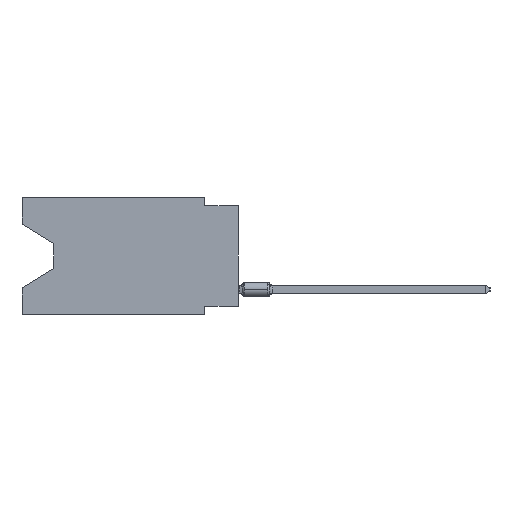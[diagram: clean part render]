
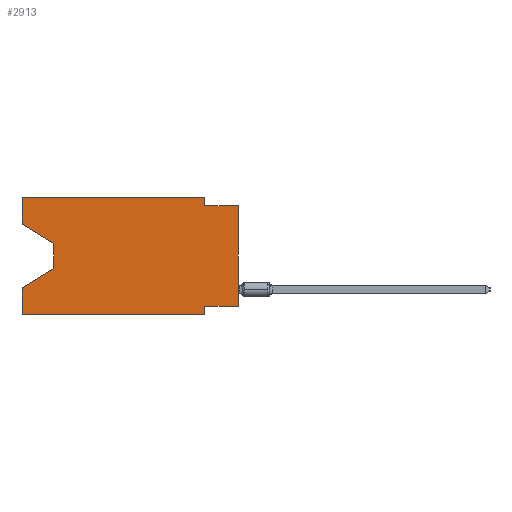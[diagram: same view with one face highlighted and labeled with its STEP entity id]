
A CAD part, left-side view. The second image highlights one B-rep face of the part: STEP entity #2913.
In plain terms, the highlighted planar face has unit normal (-1, 0, 0).
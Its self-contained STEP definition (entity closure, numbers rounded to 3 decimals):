
#907 = DIRECTION ( 'NONE',  ( 0., 0., -1. ) ) ;
#974 = CARTESIAN_POINT ( 'NONE',  ( 0., 0., 0. ) ) ;
#1068 = CARTESIAN_POINT ( 'NONE',  ( 0., 16.383, 0. ) ) ;
#1212 = VERTEX_POINT ( 'NONE', #16676 ) ;
#1256 = CARTESIAN_POINT ( 'NONE',  ( 0., 16.383, -6.852 ) ) ;
#1286 = VECTOR ( 'NONE', #34113, 1000. ) ;
#1415 = LINE ( 'NONE', #31251, #14284 ) ;
#1809 = ORIENTED_EDGE ( 'NONE', *, *, #22287, .F. ) ;
#1906 = VECTOR ( 'NONE', #17330, 1000. ) ;
#2913 = ADVANCED_FACE ( 'NONE', ( #29658 ), #21472, .F. ) ;
#3113 = ORIENTED_EDGE ( 'NONE', *, *, #12378, .F. ) ;
#3322 = CARTESIAN_POINT ( 'NONE',  ( 0., 0., -8.255 ) ) ;
#3734 = LINE ( 'NONE', #14907, #1286 ) ;
#4567 = CARTESIAN_POINT ( 'NONE',  ( 0., 16.383, 0. ) ) ;
#4703 = EDGE_CURVE ( 'NONE', #5895, #14625, #16878, .T. ) ;
#4950 = ORIENTED_EDGE ( 'NONE', *, *, #12434, .F. ) ;
#4976 = CARTESIAN_POINT ( 'NONE',  ( 0., 2.54, -8.89 ) ) ;
#5134 = CARTESIAN_POINT ( 'NONE',  ( 0., 16.383, 0. ) ) ;
#5422 = DIRECTION ( 'NONE',  ( 0., 0., 1. ) ) ;
#5499 = DIRECTION ( 'NONE',  ( 1., 0., 0. ) ) ;
#5814 = CARTESIAN_POINT ( 'NONE',  ( 0., 13.97, -5.385 ) ) ;
#5895 = VERTEX_POINT ( 'NONE', #18372 ) ;
#5934 = ORIENTED_EDGE ( 'NONE', *, *, #11839, .F. ) ;
#6814 = VERTEX_POINT ( 'NONE', #28028 ) ;
#6903 = DIRECTION ( 'NONE',  ( 0., -1., 0. ) ) ;
#7902 = CARTESIAN_POINT ( 'NONE',  ( 0., 16.383, 0. ) ) ;
#7973 = ORIENTED_EDGE ( 'NONE', *, *, #27448, .F. ) ;
#8315 = LINE ( 'NONE', #5814, #12554 ) ;
#8482 = EDGE_LOOP ( 'NONE', ( #19214, #18956, #23031, #3113, #16962, #4950, #18249, #22569, #7973, #1809, #9085, #5934 ) ) ;
#9055 = CARTESIAN_POINT ( 'NONE',  ( 0., 13.97, -3.505 ) ) ;
#9085 = ORIENTED_EDGE ( 'NONE', *, *, #10923, .F. ) ;
#9691 = DIRECTION ( 'NONE',  ( 0., -0.855, -0.519 ) ) ;
#10772 = VERTEX_POINT ( 'NONE', #22572 ) ;
#10818 = VERTEX_POINT ( 'NONE', #1256 ) ;
#10923 = EDGE_CURVE ( 'NONE', #11984, #10772, #20957, .T. ) ;
#11422 = LINE ( 'NONE', #16065, #11994 ) ;
#11678 = EDGE_CURVE ( 'NONE', #21920, #1212, #14832, .T. ) ;
#11839 = EDGE_CURVE ( 'NONE', #6814, #11984, #16071, .T. ) ;
#11984 = VERTEX_POINT ( 'NONE', #4567 ) ;
#11994 = VECTOR ( 'NONE', #27608, 1000. ) ;
#12378 = EDGE_CURVE ( 'NONE', #14106, #10818, #16700, .T. ) ;
#12434 = EDGE_CURVE ( 'NONE', #1212, #30690, #3734, .T. ) ;
#12554 = VECTOR ( 'NONE', #13980, 1000. ) ;
#12846 = VECTOR ( 'NONE', #13678, 1000. ) ;
#13065 = CARTESIAN_POINT ( 'NONE',  ( 0., 16.383, -2.038 ) ) ;
#13146 = VECTOR ( 'NONE', #33327, 1000. ) ;
#13678 = DIRECTION ( 'NONE',  ( 0., -1., 0. ) ) ;
#13980 = DIRECTION ( 'NONE',  ( 0., 0.855, -0.519 ) ) ;
#14106 = VERTEX_POINT ( 'NONE', #30367 ) ;
#14284 = VECTOR ( 'NONE', #6903, 1000. ) ;
#14577 = AXIS2_PLACEMENT_3D ( 'NONE', #5134, #5499, #18983 ) ;
#14625 = VERTEX_POINT ( 'NONE', #25851 ) ;
#14832 = LINE ( 'NONE', #33884, #1906 ) ;
#14907 = CARTESIAN_POINT ( 'NONE',  ( 0., 2.54, -8.89 ) ) ;
#16065 = CARTESIAN_POINT ( 'NONE',  ( 0., 2.54, 0. ) ) ;
#16071 = LINE ( 'NONE', #7902, #32550 ) ;
#16129 = CARTESIAN_POINT ( 'NONE',  ( 0., 2.54, -0.635 ) ) ;
#16676 = CARTESIAN_POINT ( 'NONE',  ( 0., 2.54, -8.255 ) ) ;
#16700 = LINE ( 'NONE', #1068, #25077 ) ;
#16852 = EDGE_CURVE ( 'NONE', #14106, #30690, #1415, .T. ) ;
#16878 = LINE ( 'NONE', #9055, #21626 ) ;
#16962 = ORIENTED_EDGE ( 'NONE', *, *, #16852, .T. ) ;
#16981 = VERTEX_POINT ( 'NONE', #16129 ) ;
#17117 = VECTOR ( 'NONE', #9691, 1000. ) ;
#17330 = DIRECTION ( 'NONE',  ( 0., 1., 0. ) ) ;
#18066 = EDGE_CURVE ( 'NONE', #6814, #5895, #23894, .T. ) ;
#18230 = EDGE_CURVE ( 'NONE', #21920, #29991, #30821, .T. ) ;
#18249 = ORIENTED_EDGE ( 'NONE', *, *, #11678, .F. ) ;
#18372 = CARTESIAN_POINT ( 'NONE',  ( 0., 13.97, -3.505 ) ) ;
#18956 = ORIENTED_EDGE ( 'NONE', *, *, #4703, .T. ) ;
#18983 = DIRECTION ( 'NONE',  ( 0., 0., -1. ) ) ;
#19214 = ORIENTED_EDGE ( 'NONE', *, *, #18066, .T. ) ;
#19699 = EDGE_CURVE ( 'NONE', #14625, #10818, #8315, .T. ) ;
#20957 = LINE ( 'NONE', #28425, #30336 ) ;
#21472 = PLANE ( 'NONE',  #14577 ) ;
#21626 = VECTOR ( 'NONE', #907, 1000. ) ;
#21920 = VERTEX_POINT ( 'NONE', #3322 ) ;
#22287 = EDGE_CURVE ( 'NONE', #10772, #16981, #11422, .T. ) ;
#22569 = ORIENTED_EDGE ( 'NONE', *, *, #18230, .T. ) ;
#22572 = CARTESIAN_POINT ( 'NONE',  ( 0., 2.54, 0. ) ) ;
#23031 = ORIENTED_EDGE ( 'NONE', *, *, #19699, .T. ) ;
#23894 = LINE ( 'NONE', #13065, #17117 ) ;
#24178 = LINE ( 'NONE', #35045, #12846 ) ;
#25077 = VECTOR ( 'NONE', #33770, 1000. ) ;
#25851 = CARTESIAN_POINT ( 'NONE',  ( 0., 13.97, -5.385 ) ) ;
#27448 = EDGE_CURVE ( 'NONE', #16981, #29991, #24178, .T. ) ;
#27608 = DIRECTION ( 'NONE',  ( 0., 0., -1. ) ) ;
#28028 = CARTESIAN_POINT ( 'NONE',  ( 0., 16.383, -2.038 ) ) ;
#28425 = CARTESIAN_POINT ( 'NONE',  ( 0., 16.383, 0. ) ) ;
#29658 = FACE_OUTER_BOUND ( 'NONE', #8482, .T. ) ;
#29991 = VERTEX_POINT ( 'NONE', #30092 ) ;
#30092 = CARTESIAN_POINT ( 'NONE',  ( 0., 0., -0.635 ) ) ;
#30336 = VECTOR ( 'NONE', #34503, 1000. ) ;
#30367 = CARTESIAN_POINT ( 'NONE',  ( 0., 16.383, -8.89 ) ) ;
#30690 = VERTEX_POINT ( 'NONE', #4976 ) ;
#30821 = LINE ( 'NONE', #974, #13146 ) ;
#31251 = CARTESIAN_POINT ( 'NONE',  ( 0., 16.383, -8.89 ) ) ;
#32550 = VECTOR ( 'NONE', #5422, 1000. ) ;
#33327 = DIRECTION ( 'NONE',  ( 0., 0., 1. ) ) ;
#33770 = DIRECTION ( 'NONE',  ( 0., 0., 1. ) ) ;
#33884 = CARTESIAN_POINT ( 'NONE',  ( 0., 0., -8.255 ) ) ;
#34113 = DIRECTION ( 'NONE',  ( 0., 0., -1. ) ) ;
#34503 = DIRECTION ( 'NONE',  ( 0., -1., 0. ) ) ;
#35045 = CARTESIAN_POINT ( 'NONE',  ( 0., 0., -0.635 ) ) ;
